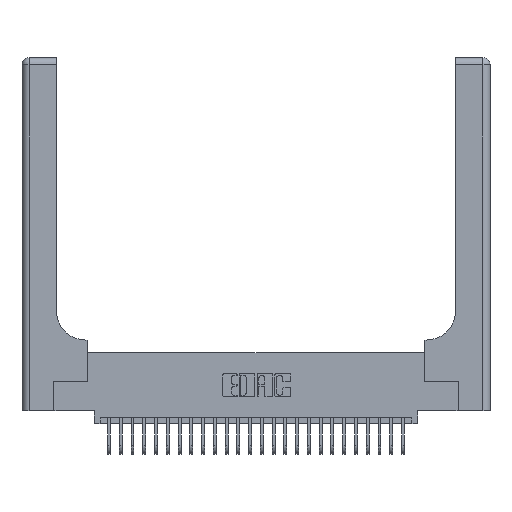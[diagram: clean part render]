
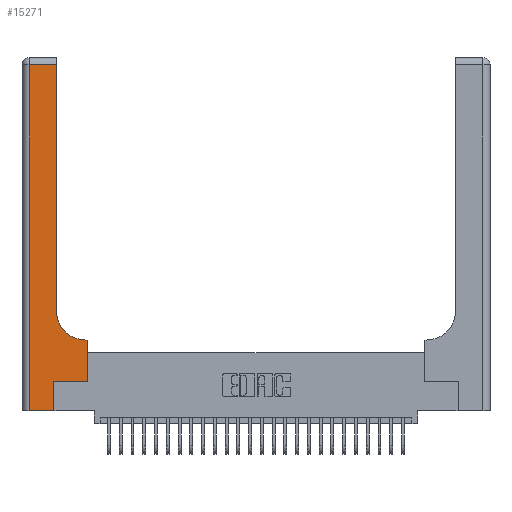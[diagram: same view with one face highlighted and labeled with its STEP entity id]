
A CAD part, top view. The second image highlights one B-rep face of the part: STEP entity #15271.
In plain terms, the highlighted planar face has unit normal (0, 0, 1).
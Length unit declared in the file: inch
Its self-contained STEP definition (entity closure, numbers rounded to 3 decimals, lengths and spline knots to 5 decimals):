
#200 = VECTOR ( 'NONE', #8582, 39.37008 ) ;
#948 = VECTOR ( 'NONE', #18202, 39.37008 ) ;
#1294 = DIRECTION ( 'NONE',  ( 1., 0., 0. ) ) ;
#2144 = VERTEX_POINT ( 'NONE', #12263 ) ;
#2705 = ORIENTED_EDGE ( 'NONE', *, *, #15150, .T. ) ;
#2756 = DIRECTION ( 'NONE',  ( 0., -1., 0. ) ) ;
#2775 = ORIENTED_EDGE ( 'NONE', *, *, #4064, .T. ) ;
#2821 = VECTOR ( 'NONE', #1294, 39.37008 ) ;
#3028 = DIRECTION ( 'NONE',  ( -1., 0., 0. ) ) ;
#3052 = CARTESIAN_POINT ( 'NONE',  ( 0.5415, 0.85, 0.37 ) ) ;
#3530 = VECTOR ( 'NONE', #18932, 39.37008 ) ;
#3876 = CARTESIAN_POINT ( 'NONE',  ( 0.5415, 0.6, 0.37 ) ) ;
#3975 = CARTESIAN_POINT ( 'NONE',  ( 0.06, 2.94, 0.37 ) ) ;
#4064 = EDGE_CURVE ( 'NONE', #7580, #6164, #16037, .T. ) ;
#4370 = CARTESIAN_POINT ( 'NONE',  ( 0.269, 0.25, 0.37 ) ) ;
#5050 = ORIENTED_EDGE ( 'NONE', *, *, #23755, .T. ) ;
#5141 = DIRECTION ( 'NONE',  ( 1., 0., 0. ) ) ;
#5568 = CIRCLE ( 'NONE', #19431, 0.25 ) ;
#5722 = EDGE_CURVE ( 'NONE', #13094, #6145, #21843, .T. ) ;
#6145 = VERTEX_POINT ( 'NONE', #3876 ) ;
#6164 = VERTEX_POINT ( 'NONE', #3975 ) ;
#6288 = EDGE_CURVE ( 'NONE', #15003, #13094, #9100, .T. ) ;
#6302 = ORIENTED_EDGE ( 'NONE', *, *, #26102, .T. ) ;
#6477 = LINE ( 'NONE', #4370, #200 ) ;
#6529 = LINE ( 'NONE', #7819, #948 ) ;
#6586 = CARTESIAN_POINT ( 'NONE',  ( 0., 2.94, 0.37 ) ) ;
#6645 = CARTESIAN_POINT ( 'NONE',  ( 0.2915, 0.6, 0.37 ) ) ;
#6762 = PLANE ( 'NONE',  #13770 ) ;
#6989 = CARTESIAN_POINT ( 'NONE',  ( 0.5585, 0.6, 0.37 ) ) ;
#7580 = VERTEX_POINT ( 'NONE', #12939 ) ;
#7819 = CARTESIAN_POINT ( 'NONE',  ( 0.2915, 3., 0.37 ) ) ;
#8045 = CARTESIAN_POINT ( 'NONE',  ( 0.5585, 0.25, 0.37 ) ) ;
#8382 = LINE ( 'NONE', #17895, #2821 ) ;
#8529 = CARTESIAN_POINT ( 'NONE',  ( 0.5585, 0.25, 0.37 ) ) ;
#8569 = CARTESIAN_POINT ( 'NONE',  ( 0.269, 0., 0.37 ) ) ;
#8582 = DIRECTION ( 'NONE',  ( 1., 0., 0. ) ) ;
#9100 = LINE ( 'NONE', #8529, #3530 ) ;
#9908 = CARTESIAN_POINT ( 'NONE',  ( 0.06, 0., 0.37 ) ) ;
#11275 = ORIENTED_EDGE ( 'NONE', *, *, #5722, .T. ) ;
#11851 = VECTOR ( 'NONE', #21160, 39.37008 ) ;
#12226 = LINE ( 'NONE', #13156, #17071 ) ;
#12263 = CARTESIAN_POINT ( 'NONE',  ( 0.269, 0., 0.37 ) ) ;
#12588 = ORIENTED_EDGE ( 'NONE', *, *, #14254, .T. ) ;
#12939 = CARTESIAN_POINT ( 'NONE',  ( 0.2915, 2.94, 0.37 ) ) ;
#13094 = VERTEX_POINT ( 'NONE', #6989 ) ;
#13156 = CARTESIAN_POINT ( 'NONE',  ( 0.06, 3., 0.37 ) ) ;
#13770 = AXIS2_PLACEMENT_3D ( 'NONE', #19242, #15475, #3028 ) ;
#14254 = EDGE_CURVE ( 'NONE', #24136, #7580, #6529, .T. ) ;
#14841 = DIRECTION ( 'NONE',  ( 0., 1., 0. ) ) ;
#15003 = VERTEX_POINT ( 'NONE', #8045 ) ;
#15150 = EDGE_CURVE ( 'NONE', #19241, #15003, #6477, .T. ) ;
#15271 = ADVANCED_FACE ( 'NONE', ( #19831 ), #6762, .F. ) ;
#15475 = DIRECTION ( 'NONE',  ( 0., 0., -1. ) ) ;
#16037 = LINE ( 'NONE', #6586, #11851 ) ;
#16776 = ORIENTED_EDGE ( 'NONE', *, *, #19768, .T. ) ;
#16929 = VECTOR ( 'NONE', #21221, 39.37008 ) ;
#17057 = EDGE_LOOP ( 'NONE', ( #12588, #2775, #6302, #5050, #16776, #2705, #17460, #11275, #18720 ) ) ;
#17071 = VECTOR ( 'NONE', #2756, 39.37008 ) ;
#17460 = ORIENTED_EDGE ( 'NONE', *, *, #6288, .T. ) ;
#17631 = DIRECTION ( 'NONE',  ( 0., 0., -1. ) ) ;
#17895 = CARTESIAN_POINT ( 'NONE',  ( 0., 0., 0.37 ) ) ;
#18202 = DIRECTION ( 'NONE',  ( 0., 1., 0. ) ) ;
#18340 = LINE ( 'NONE', #8569, #23211 ) ;
#18720 = ORIENTED_EDGE ( 'NONE', *, *, #20483, .T. ) ;
#18932 = DIRECTION ( 'NONE',  ( 0., 1., 0. ) ) ;
#19241 = VERTEX_POINT ( 'NONE', #20302 ) ;
#19242 = CARTESIAN_POINT ( 'NONE',  ( 0., 3., 0.37 ) ) ;
#19431 = AXIS2_PLACEMENT_3D ( 'NONE', #3052, #17631, #5141 ) ;
#19519 = CARTESIAN_POINT ( 'NONE',  ( 0.2915, 0.85, 0.37 ) ) ;
#19768 = EDGE_CURVE ( 'NONE', #2144, #19241, #18340, .T. ) ;
#19831 = FACE_OUTER_BOUND ( 'NONE', #17057, .T. ) ;
#20302 = CARTESIAN_POINT ( 'NONE',  ( 0.269, 0.25, 0.37 ) ) ;
#20483 = EDGE_CURVE ( 'NONE', #6145, #24136, #5568, .T. ) ;
#20671 = VERTEX_POINT ( 'NONE', #9908 ) ;
#21160 = DIRECTION ( 'NONE',  ( -1., 0., 0. ) ) ;
#21221 = DIRECTION ( 'NONE',  ( -1., 0., 0. ) ) ;
#21843 = LINE ( 'NONE', #6645, #16929 ) ;
#23211 = VECTOR ( 'NONE', #14841, 39.37008 ) ;
#23755 = EDGE_CURVE ( 'NONE', #20671, #2144, #8382, .T. ) ;
#24136 = VERTEX_POINT ( 'NONE', #19519 ) ;
#26102 = EDGE_CURVE ( 'NONE', #6164, #20671, #12226, .T. ) ;
